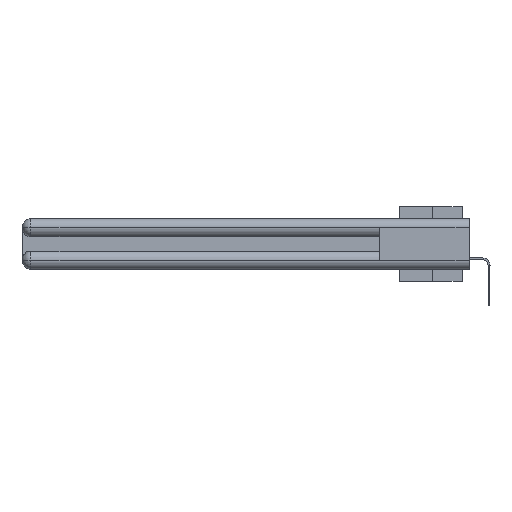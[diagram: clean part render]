
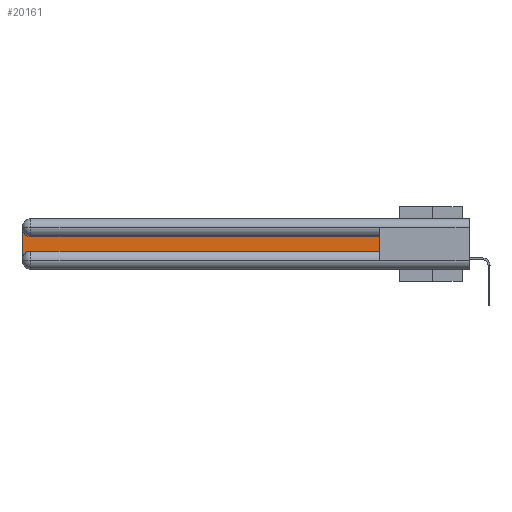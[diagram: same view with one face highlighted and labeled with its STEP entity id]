
A CAD part, left-side view. The second image highlights one B-rep face of the part: STEP entity #20161.
In plain terms, the highlighted planar face has unit normal (-1, 0, 0).
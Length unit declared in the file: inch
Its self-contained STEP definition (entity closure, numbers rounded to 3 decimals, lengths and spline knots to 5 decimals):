
#607 = CARTESIAN_POINT ( 'NONE',  ( 0.075, 2.94, -0.2775 ) ) ;
#1266 = CIRCLE ( 'NONE', #3177, 0.06 ) ;
#1323 = AXIS2_PLACEMENT_3D ( 'NONE', #607, #7189, #25950 ) ;
#3177 = AXIS2_PLACEMENT_3D ( 'NONE', #29054, #26934, #10615 ) ;
#3474 = CARTESIAN_POINT ( 'NONE',  ( 0.075, 0.6, -0.2175 ) ) ;
#4073 = ORIENTED_EDGE ( 'NONE', *, *, #8713, .T. ) ;
#5640 = EDGE_LOOP ( 'NONE', ( #27242, #15412, #13352, #7712, #4073, #21433 ) ) ;
#6292 = CARTESIAN_POINT ( 'NONE',  ( 0.075, 3., -0.2775 ) ) ;
#6715 = VERTEX_POINT ( 'NONE', #12738 ) ;
#7189 = DIRECTION ( 'NONE',  ( 1., 0., 0. ) ) ;
#7712 = ORIENTED_EDGE ( 'NONE', *, *, #16441, .T. ) ;
#8066 = DIRECTION ( 'NONE',  ( 0., -1., 0. ) ) ;
#8237 = DIRECTION ( 'NONE',  ( 0., 0., -1. ) ) ;
#8713 = EDGE_CURVE ( 'NONE', #6715, #27613, #29197, .T. ) ;
#8871 = CARTESIAN_POINT ( 'NONE',  ( 0.075, 0.6, -0.1225 ) ) ;
#10615 = DIRECTION ( 'NONE',  ( 0., 0., -1. ) ) ;
#10626 = DIRECTION ( 'NONE',  ( 0., 0., 1. ) ) ;
#10764 = LINE ( 'NONE', #26577, #16542 ) ;
#10800 = VERTEX_POINT ( 'NONE', #17030 ) ;
#10942 = CARTESIAN_POINT ( 'NONE',  ( 0.075, 0.6, -0.1225 ) ) ;
#10995 = EDGE_CURVE ( 'NONE', #10800, #11944, #10764, .T. ) ;
#11165 = CIRCLE ( 'NONE', #1323, 0.06 ) ;
#11266 = LINE ( 'NONE', #29163, #15250 ) ;
#11442 = VERTEX_POINT ( 'NONE', #8871 ) ;
#11520 = LINE ( 'NONE', #10942, #15871 ) ;
#11944 = VERTEX_POINT ( 'NONE', #6292 ) ;
#12375 = CARTESIAN_POINT ( 'NONE',  ( 0.075, 3., -0.1225 ) ) ;
#12738 = CARTESIAN_POINT ( 'NONE',  ( 0.075, 2.94, -0.2175 ) ) ;
#13054 = EDGE_CURVE ( 'NONE', #24676, #10800, #1266, .T. ) ;
#13260 = DIRECTION ( 'NONE',  ( 0., 1., 0. ) ) ;
#13352 = ORIENTED_EDGE ( 'NONE', *, *, #10995, .T. ) ;
#15250 = VECTOR ( 'NONE', #10626, 39.37008 ) ;
#15412 = ORIENTED_EDGE ( 'NONE', *, *, #13054, .T. ) ;
#15871 = VECTOR ( 'NONE', #13260, 39.37008 ) ;
#16385 = FACE_OUTER_BOUND ( 'NONE', #5640, .T. ) ;
#16441 = EDGE_CURVE ( 'NONE', #11944, #6715, #11165, .T. ) ;
#16542 = VECTOR ( 'NONE', #8237, 39.37008 ) ;
#17030 = CARTESIAN_POINT ( 'NONE',  ( 0.075, 3., -0.0625 ) ) ;
#17251 = EDGE_CURVE ( 'NONE', #11442, #24676, #11520, .T. ) ;
#19428 = DIRECTION ( 'NONE',  ( 1., 0., 0. ) ) ;
#20161 = ADVANCED_FACE ( 'NONE', ( #16385 ), #28692, .F. ) ;
#20559 = VECTOR ( 'NONE', #8066, 39.37008 ) ;
#21433 = ORIENTED_EDGE ( 'NONE', *, *, #24819, .T. ) ;
#24676 = VERTEX_POINT ( 'NONE', #26062 ) ;
#24819 = EDGE_CURVE ( 'NONE', #27613, #11442, #11266, .T. ) ;
#25950 = DIRECTION ( 'NONE',  ( 0., 0., -1. ) ) ;
#26062 = CARTESIAN_POINT ( 'NONE',  ( 0.075, 2.94, -0.1225 ) ) ;
#26577 = CARTESIAN_POINT ( 'NONE',  ( 0.075, 3., -0.2175 ) ) ;
#26934 = DIRECTION ( 'NONE',  ( 1., 0., 0. ) ) ;
#27242 = ORIENTED_EDGE ( 'NONE', *, *, #17251, .T. ) ;
#27613 = VERTEX_POINT ( 'NONE', #27977 ) ;
#27977 = CARTESIAN_POINT ( 'NONE',  ( 0.075, 0.6, -0.2175 ) ) ;
#28692 = PLANE ( 'NONE',  #29037 ) ;
#28792 = DIRECTION ( 'NONE',  ( 0., 0., -1. ) ) ;
#29037 = AXIS2_PLACEMENT_3D ( 'NONE', #12375, #19428, #28792 ) ;
#29054 = CARTESIAN_POINT ( 'NONE',  ( 0.075, 2.94, -0.0625 ) ) ;
#29163 = CARTESIAN_POINT ( 'NONE',  ( 0.075, 0.6, -0.2175 ) ) ;
#29197 = LINE ( 'NONE', #3474, #20559 ) ;
